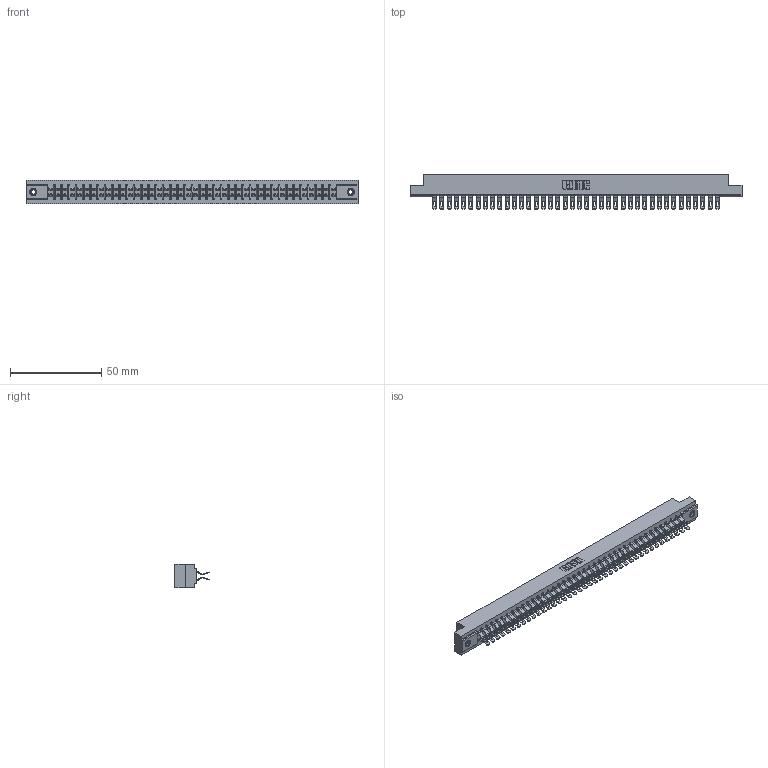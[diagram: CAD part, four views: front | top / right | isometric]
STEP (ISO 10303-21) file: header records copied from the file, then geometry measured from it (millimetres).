
FILE_DESCRIPTION (( 'STEP AP203' ), '1' );
FILE_NAME ('357-080-455-207.STEP', '2020-10-04T11:30:19', ( '' ), ( '' ), 'SwSTEP 2.0', 'SolidWorks 2020', '' );
FILE_SCHEMA (( 'CONFIG_CONTROL_DESIGN' ));
Length unit declared in the file: inch
Products named in the file (4): 307 Part_.156 Dia Mounting Holes; 307-290-001_555; 357-080-455-207; 345-250-001_345-250-005-103
Assembly tree (83 placements, depth 2):
  357-080-455-207
    307 Part_.156 Dia Mounting Holes
    307-290-001_555  x80
    345-250-001_345-250-005-103  x2
Bounding box: 181.51 x 18.75 x 12.7 mm (x, y, z)
Volume: 19511.9 mm3; surface area: 25189.8 mm2
Topology: 83 solids, 83 shells, 5099 faces, 14939 edges, 9734 vertices
Faces by surface type: plane 2822, cylinder 2179, sphere 82, cone 12, torus 4
Entity records: 37540 total; most frequent: CARTESIAN_POINT 6131, ORIENTED_EDGE 6072, DIRECTION 6022, EDGE_CURVE 3036, VECTOR 2316, LINE 2316, VERTEX_POINT 1962, AXIS2_PLACEMENT_3D 1853
